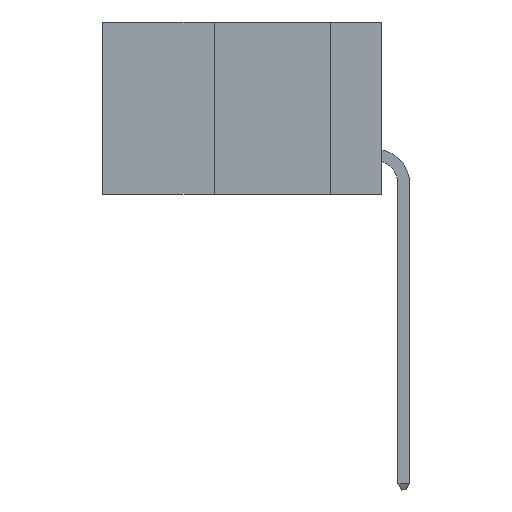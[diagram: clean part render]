
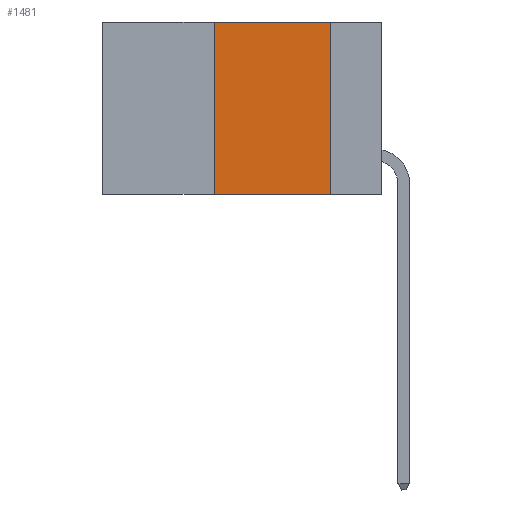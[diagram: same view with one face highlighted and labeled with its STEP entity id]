
A CAD part, left-side view. The second image highlights one B-rep face of the part: STEP entity #1481.
In plain terms, the highlighted planar face has unit normal (-1, 0, 0).
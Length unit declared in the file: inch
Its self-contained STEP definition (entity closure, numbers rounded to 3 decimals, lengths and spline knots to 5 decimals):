
#949 = LINE ( 'NONE', #21436, #31981 ) ;
#1210 = VECTOR ( 'NONE', #41077, 39.37008 ) ;
#1481 = ADVANCED_FACE ( 'NONE', ( #8037 ), #42502, .F. ) ;
#4791 = CARTESIAN_POINT ( 'NONE',  ( 0., 0.11, 0. ) ) ;
#6180 = VERTEX_POINT ( 'NONE', #18939 ) ;
#6373 = AXIS2_PLACEMENT_3D ( 'NONE', #39367, #12035, #11591 ) ;
#6442 = CARTESIAN_POINT ( 'NONE',  ( 0., 0.36, -0.37 ) ) ;
#7147 = EDGE_LOOP ( 'NONE', ( #35520, #29834, #8570, #19431 ) ) ;
#8037 = FACE_OUTER_BOUND ( 'NONE', #7147, .T. ) ;
#8292 = VECTOR ( 'NONE', #15026, 39.37008 ) ;
#8570 = ORIENTED_EDGE ( 'NONE', *, *, #33317, .F. ) ;
#9958 = CARTESIAN_POINT ( 'NONE',  ( 0., 0.6, -0.37 ) ) ;
#11591 = DIRECTION ( 'NONE',  ( 0., 0., -1. ) ) ;
#12035 = DIRECTION ( 'NONE',  ( 1., 0., 0. ) ) ;
#12047 = VERTEX_POINT ( 'NONE', #6442 ) ;
#15026 = DIRECTION ( 'NONE',  ( 0., 0., -1. ) ) ;
#15285 = VERTEX_POINT ( 'NONE', #25612 ) ;
#15915 = EDGE_CURVE ( 'NONE', #12047, #6180, #20190, .T. ) ;
#18939 = CARTESIAN_POINT ( 'NONE',  ( 0., 0.11, -0.37 ) ) ;
#19431 = ORIENTED_EDGE ( 'NONE', *, *, #15915, .T. ) ;
#20190 = LINE ( 'NONE', #9958, #1210 ) ;
#21436 = CARTESIAN_POINT ( 'NONE',  ( 0., 0.6, 0. ) ) ;
#25307 = CARTESIAN_POINT ( 'NONE',  ( 0., 0.36, 0. ) ) ;
#25612 = CARTESIAN_POINT ( 'NONE',  ( 0., 0.11, 0. ) ) ;
#25859 = CARTESIAN_POINT ( 'NONE',  ( 0., 0.36, 0. ) ) ;
#27720 = LINE ( 'NONE', #4791, #8292 ) ;
#28616 = VECTOR ( 'NONE', #39409, 39.37008 ) ;
#29193 = LINE ( 'NONE', #25859, #28616 ) ;
#29834 = ORIENTED_EDGE ( 'NONE', *, *, #30494, .F. ) ;
#30494 = EDGE_CURVE ( 'NONE', #40904, #15285, #949, .T. ) ;
#31981 = VECTOR ( 'NONE', #41886, 39.37008 ) ;
#33317 = EDGE_CURVE ( 'NONE', #12047, #40904, #29193, .T. ) ;
#35520 = ORIENTED_EDGE ( 'NONE', *, *, #41369, .F. ) ;
#39367 = CARTESIAN_POINT ( 'NONE',  ( 0., 0.6, 0. ) ) ;
#39409 = DIRECTION ( 'NONE',  ( 0., 0., 1. ) ) ;
#40904 = VERTEX_POINT ( 'NONE', #25307 ) ;
#41077 = DIRECTION ( 'NONE',  ( 0., -1., 0. ) ) ;
#41369 = EDGE_CURVE ( 'NONE', #15285, #6180, #27720, .T. ) ;
#41886 = DIRECTION ( 'NONE',  ( 0., -1., 0. ) ) ;
#42502 = PLANE ( 'NONE',  #6373 ) ;
